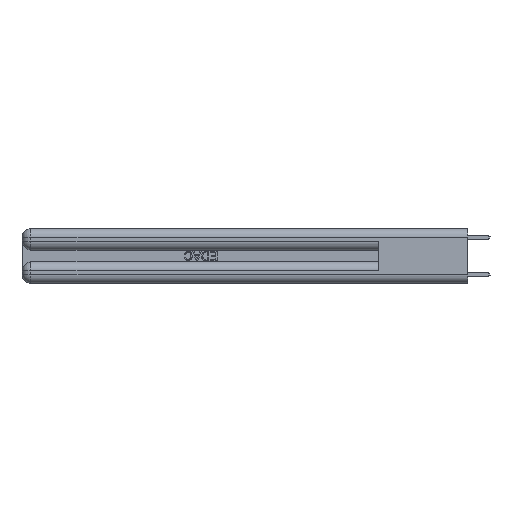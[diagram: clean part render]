
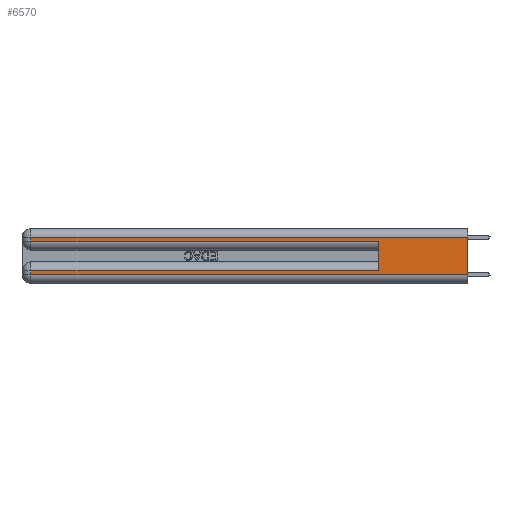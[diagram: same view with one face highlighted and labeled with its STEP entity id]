
A CAD part, left-side view. The second image highlights one B-rep face of the part: STEP entity #6570.
In plain terms, the highlighted planar face has unit normal (-1, 0, 0).
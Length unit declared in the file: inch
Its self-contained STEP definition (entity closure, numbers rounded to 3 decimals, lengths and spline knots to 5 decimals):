
#473 = DIRECTION ( 'NONE',  ( 1., 0., 0. ) ) ;
#1189 = VERTEX_POINT ( 'NONE', #4638 ) ;
#1262 = ORIENTED_EDGE ( 'NONE', *, *, #22873, .T. ) ;
#1520 = VERTEX_POINT ( 'NONE', #20198 ) ;
#3409 = CARTESIAN_POINT ( 'NONE',  ( 0., 2.94, 0.085 ) ) ;
#3686 = CARTESIAN_POINT ( 'NONE',  ( 0., 0.6, 0.285 ) ) ;
#3692 = CARTESIAN_POINT ( 'NONE',  ( 0., 0., 0.31 ) ) ;
#4385 = DIRECTION ( 'NONE',  ( 0., 0., -1. ) ) ;
#4638 = CARTESIAN_POINT ( 'NONE',  ( 0., 2.94, 0.285 ) ) ;
#5492 = LINE ( 'NONE', #21988, #7699 ) ;
#6570 = ADVANCED_FACE ( 'NONE', ( #27920 ), #14123, .F. ) ;
#6748 = CARTESIAN_POINT ( 'NONE',  ( 0., 0., 0.06 ) ) ;
#7162 = DIRECTION ( 'NONE',  ( 0., 0., -1. ) ) ;
#7602 = EDGE_CURVE ( 'NONE', #23822, #17461, #21616, .T. ) ;
#7680 = CARTESIAN_POINT ( 'NONE',  ( 0., 2.94, 0.37 ) ) ;
#7699 = VECTOR ( 'NONE', #10339, 39.37008 ) ;
#8359 = CARTESIAN_POINT ( 'NONE',  ( 0., 2.94, 0.31 ) ) ;
#8566 = DIRECTION ( 'NONE',  ( 0., -1., 0. ) ) ;
#9514 = LINE ( 'NONE', #25138, #29392 ) ;
#9973 = CARTESIAN_POINT ( 'NONE',  ( 0., 0., 0.085 ) ) ;
#10280 = LINE ( 'NONE', #9973, #12987 ) ;
#10339 = DIRECTION ( 'NONE',  ( 0., 0., 1. ) ) ;
#12277 = ORIENTED_EDGE ( 'NONE', *, *, #12313, .T. ) ;
#12313 = EDGE_CURVE ( 'NONE', #1189, #21643, #26629, .T. ) ;
#12987 = VECTOR ( 'NONE', #26060, 39.37008 ) ;
#13032 = ORIENTED_EDGE ( 'NONE', *, *, #23595, .F. ) ;
#13811 = CARTESIAN_POINT ( 'NONE',  ( 0., 0., 0.37 ) ) ;
#14123 = PLANE ( 'NONE',  #18748 ) ;
#14763 = VECTOR ( 'NONE', #22162, 39.37008 ) ;
#15192 = ORIENTED_EDGE ( 'NONE', *, *, #16359, .T. ) ;
#15443 = VERTEX_POINT ( 'NONE', #27541 ) ;
#15973 = DIRECTION ( 'NONE',  ( 0., -1., 0. ) ) ;
#16359 = EDGE_CURVE ( 'NONE', #18013, #23822, #10280, .T. ) ;
#17461 = VERTEX_POINT ( 'NONE', #24731 ) ;
#17669 = EDGE_LOOP ( 'NONE', ( #13032, #1262, #25355, #12277, #19646, #15192, #20437, #22795 ) ) ;
#18013 = VERTEX_POINT ( 'NONE', #20707 ) ;
#18221 = LINE ( 'NONE', #6748, #29689 ) ;
#18748 = AXIS2_PLACEMENT_3D ( 'NONE', #13811, #473, #7162 ) ;
#18869 = DIRECTION ( 'NONE',  ( 0., 0., -1. ) ) ;
#19646 = ORIENTED_EDGE ( 'NONE', *, *, #24356, .F. ) ;
#20198 = CARTESIAN_POINT ( 'NONE',  ( 0., 0., 0.31 ) ) ;
#20410 = VECTOR ( 'NONE', #8566, 39.37008 ) ;
#20437 = ORIENTED_EDGE ( 'NONE', *, *, #7602, .T. ) ;
#20707 = CARTESIAN_POINT ( 'NONE',  ( 0., 0.6, 0.085 ) ) ;
#21616 = LINE ( 'NONE', #7680, #25139 ) ;
#21643 = VERTEX_POINT ( 'NONE', #3686 ) ;
#21988 = CARTESIAN_POINT ( 'NONE',  ( 0., 0.6, 0.145 ) ) ;
#22096 = LINE ( 'NONE', #26526, #29448 ) ;
#22162 = DIRECTION ( 'NONE',  ( 0., 1., 0. ) ) ;
#22247 = DIRECTION ( 'NONE',  ( 0., 0., -1. ) ) ;
#22795 = ORIENTED_EDGE ( 'NONE', *, *, #27329, .T. ) ;
#22873 = EDGE_CURVE ( 'NONE', #1520, #27869, #23976, .T. ) ;
#23595 = EDGE_CURVE ( 'NONE', #1520, #15443, #22096, .T. ) ;
#23822 = VERTEX_POINT ( 'NONE', #3409 ) ;
#23976 = LINE ( 'NONE', #3692, #14763 ) ;
#24356 = EDGE_CURVE ( 'NONE', #18013, #21643, #5492, .T. ) ;
#24731 = CARTESIAN_POINT ( 'NONE',  ( 0., 2.94, 0.06 ) ) ;
#25138 = CARTESIAN_POINT ( 'NONE',  ( 0., 2.94, 0.37 ) ) ;
#25139 = VECTOR ( 'NONE', #18869, 39.37008 ) ;
#25355 = ORIENTED_EDGE ( 'NONE', *, *, #26481, .T. ) ;
#26060 = DIRECTION ( 'NONE',  ( 0., 1., 0. ) ) ;
#26481 = EDGE_CURVE ( 'NONE', #27869, #1189, #9514, .T. ) ;
#26526 = CARTESIAN_POINT ( 'NONE',  ( 0., 0., 0.37 ) ) ;
#26629 = LINE ( 'NONE', #26772, #20410 ) ;
#26772 = CARTESIAN_POINT ( 'NONE',  ( 0., 0., 0.285 ) ) ;
#27329 = EDGE_CURVE ( 'NONE', #17461, #15443, #18221, .T. ) ;
#27541 = CARTESIAN_POINT ( 'NONE',  ( 0., 0., 0.06 ) ) ;
#27869 = VERTEX_POINT ( 'NONE', #8359 ) ;
#27920 = FACE_OUTER_BOUND ( 'NONE', #17669, .T. ) ;
#29392 = VECTOR ( 'NONE', #4385, 39.37008 ) ;
#29448 = VECTOR ( 'NONE', #22247, 39.37008 ) ;
#29689 = VECTOR ( 'NONE', #15973, 39.37008 ) ;
